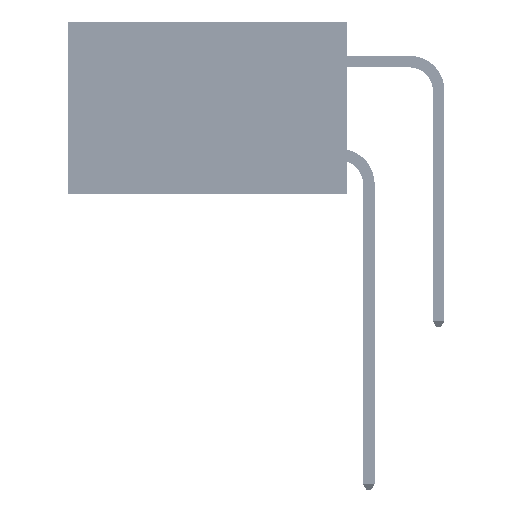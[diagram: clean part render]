
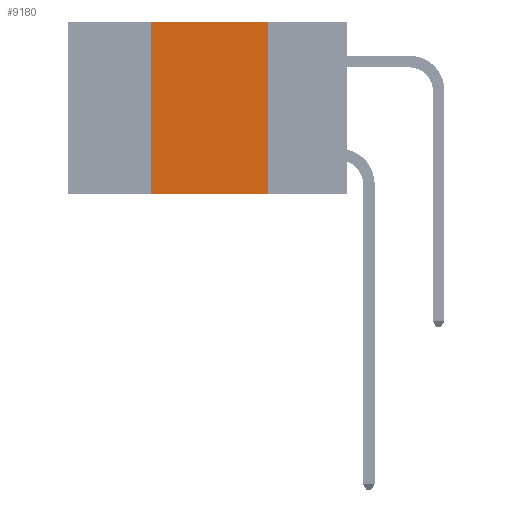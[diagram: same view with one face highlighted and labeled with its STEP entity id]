
A CAD part, left-side view. The second image highlights one B-rep face of the part: STEP entity #9180.
In plain terms, the highlighted planar face has unit normal (-1, 0, 0).
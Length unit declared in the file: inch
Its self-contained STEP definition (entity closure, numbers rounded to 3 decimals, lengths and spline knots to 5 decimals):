
#2328 = CARTESIAN_POINT ( 'NONE',  ( 0., 0.42, 0. ) ) ;
#4136 = VERTEX_POINT ( 'NONE', #31434 ) ;
#4225 = PLANE ( 'NONE',  #42478 ) ;
#6159 = CARTESIAN_POINT ( 'NONE',  ( 0., 0.42, -0.37 ) ) ;
#8845 = CARTESIAN_POINT ( 'NONE',  ( 0., 0.6, 0. ) ) ;
#8998 = VERTEX_POINT ( 'NONE', #52986 ) ;
#9128 = VECTOR ( 'NONE', #27303, 39.37008 ) ;
#9180 = ADVANCED_FACE ( 'NONE', ( #23304 ), #4225, .F. ) ;
#10314 = LINE ( 'NONE', #2328, #49665 ) ;
#14590 = DIRECTION ( 'NONE',  ( 0., 0., 1. ) ) ;
#20305 = LINE ( 'NONE', #23631, #9128 ) ;
#21087 = DIRECTION ( 'NONE',  ( 1., 0., 0. ) ) ;
#22106 = ORIENTED_EDGE ( 'NONE', *, *, #39810, .T. ) ;
#23304 = FACE_OUTER_BOUND ( 'NONE', #43904, .T. ) ;
#23631 = CARTESIAN_POINT ( 'NONE',  ( 0., 0.6, -0.37 ) ) ;
#25320 = CARTESIAN_POINT ( 'NONE',  ( 0., 0.6, 0. ) ) ;
#26418 = EDGE_CURVE ( 'NONE', #41653, #8998, #10314, .T. ) ;
#26975 = CARTESIAN_POINT ( 'NONE',  ( 0., 0.17, -0.37 ) ) ;
#27303 = DIRECTION ( 'NONE',  ( 0., -1., 0. ) ) ;
#29156 = DIRECTION ( 'NONE',  ( 0., 0., -1. ) ) ;
#29946 = DIRECTION ( 'NONE',  ( 0., -1., 0. ) ) ;
#30294 = VECTOR ( 'NONE', #49599, 39.37008 ) ;
#31245 = VERTEX_POINT ( 'NONE', #26975 ) ;
#31434 = CARTESIAN_POINT ( 'NONE',  ( 0., 0.17, 0. ) ) ;
#32008 = ORIENTED_EDGE ( 'NONE', *, *, #33161, .F. ) ;
#33161 = EDGE_CURVE ( 'NONE', #4136, #31245, #42770, .T. ) ;
#33738 = ORIENTED_EDGE ( 'NONE', *, *, #26418, .F. ) ;
#35690 = ORIENTED_EDGE ( 'NONE', *, *, #38830, .F. ) ;
#37011 = CARTESIAN_POINT ( 'NONE',  ( 0., 0.17, 0. ) ) ;
#38830 = EDGE_CURVE ( 'NONE', #8998, #4136, #46018, .T. ) ;
#39810 = EDGE_CURVE ( 'NONE', #41653, #31245, #20305, .T. ) ;
#41653 = VERTEX_POINT ( 'NONE', #6159 ) ;
#42478 = AXIS2_PLACEMENT_3D ( 'NONE', #25320, #21087, #29156 ) ;
#42770 = LINE ( 'NONE', #37011, #30294 ) ;
#43904 = EDGE_LOOP ( 'NONE', ( #32008, #35690, #33738, #22106 ) ) ;
#46018 = LINE ( 'NONE', #8845, #48651 ) ;
#48651 = VECTOR ( 'NONE', #29946, 39.37008 ) ;
#49599 = DIRECTION ( 'NONE',  ( 0., 0., -1. ) ) ;
#49665 = VECTOR ( 'NONE', #14590, 39.37008 ) ;
#52986 = CARTESIAN_POINT ( 'NONE',  ( 0., 0.42, 0. ) ) ;
